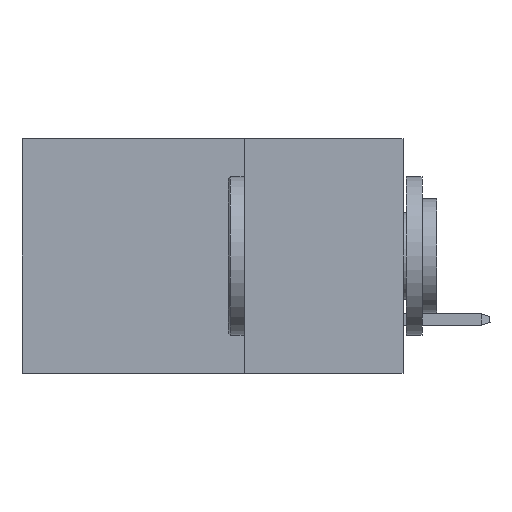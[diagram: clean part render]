
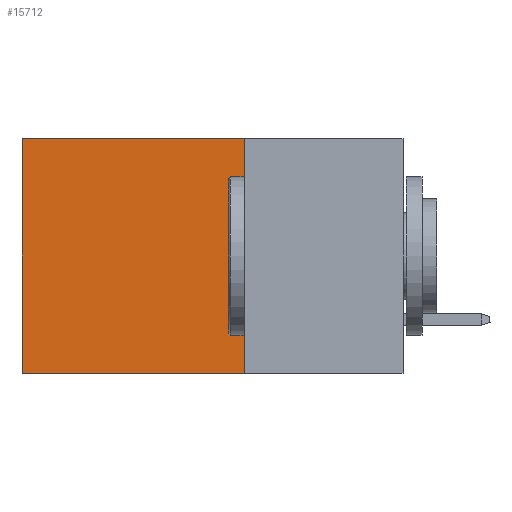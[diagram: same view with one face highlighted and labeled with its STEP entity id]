
A CAD part, left-side view. The second image highlights one B-rep face of the part: STEP entity #15712.
In plain terms, the highlighted planar face has unit normal (-1, 0, 0).
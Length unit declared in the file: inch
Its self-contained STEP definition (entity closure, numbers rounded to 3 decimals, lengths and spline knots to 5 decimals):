
#242 = LINE ( 'NONE', #23658, #15980 ) ;
#714 = VERTEX_POINT ( 'NONE', #7614 ) ;
#3190 = LINE ( 'NONE', #23038, #6921 ) ;
#3958 = VERTEX_POINT ( 'NONE', #17272 ) ;
#5454 = CARTESIAN_POINT ( 'NONE',  ( 0.2875, 0.25, 0. ) ) ;
#5765 = CARTESIAN_POINT ( 'NONE',  ( 0.2875, 0.25, 0. ) ) ;
#5849 = DIRECTION ( 'NONE',  ( 0., 0., -1. ) ) ;
#6921 = VECTOR ( 'NONE', #5849, 39.37008 ) ;
#7309 = EDGE_CURVE ( 'NONE', #17870, #3958, #10928, .T. ) ;
#7534 = EDGE_CURVE ( 'NONE', #3958, #714, #3190, .T. ) ;
#7614 = CARTESIAN_POINT ( 'NONE',  ( 0.2875, 0.6, -0.37 ) ) ;
#10928 = LINE ( 'NONE', #22209, #21706 ) ;
#11769 = EDGE_CURVE ( 'NONE', #17870, #19024, #21649, .T. ) ;
#11937 = ORIENTED_EDGE ( 'NONE', *, *, #7309, .T. ) ;
#12042 = ORIENTED_EDGE ( 'NONE', *, *, #7534, .T. ) ;
#12788 = DIRECTION ( 'NONE',  ( 1., 0., 0. ) ) ;
#14540 = AXIS2_PLACEMENT_3D ( 'NONE', #5765, #12788, #22839 ) ;
#15059 = CARTESIAN_POINT ( 'NONE',  ( 0.2875, 0.25, 0. ) ) ;
#15712 = ADVANCED_FACE ( 'NONE', ( #15724 ), #25125, .F. ) ;
#15724 = FACE_OUTER_BOUND ( 'NONE', #30210, .T. ) ;
#15980 = VECTOR ( 'NONE', #21356, 39.37008 ) ;
#16166 = EDGE_CURVE ( 'NONE', #19024, #714, #242, .T. ) ;
#17272 = CARTESIAN_POINT ( 'NONE',  ( 0.2875, 0.6, 0. ) ) ;
#17870 = VERTEX_POINT ( 'NONE', #15059 ) ;
#18013 = DIRECTION ( 'NONE',  ( 0., 1., 0. ) ) ;
#19024 = VERTEX_POINT ( 'NONE', #30000 ) ;
#19863 = ORIENTED_EDGE ( 'NONE', *, *, #11769, .F. ) ;
#21356 = DIRECTION ( 'NONE',  ( 0., 1., 0. ) ) ;
#21649 = LINE ( 'NONE', #5454, #21797 ) ;
#21706 = VECTOR ( 'NONE', #18013, 39.37008 ) ;
#21797 = VECTOR ( 'NONE', #24550, 39.37008 ) ;
#22209 = CARTESIAN_POINT ( 'NONE',  ( 0.2875, 0.25, 0. ) ) ;
#22839 = DIRECTION ( 'NONE',  ( 0., 0., -1. ) ) ;
#23038 = CARTESIAN_POINT ( 'NONE',  ( 0.2875, 0.6, 0. ) ) ;
#23658 = CARTESIAN_POINT ( 'NONE',  ( 0.2875, 0.25, -0.37 ) ) ;
#24550 = DIRECTION ( 'NONE',  ( 0., 0., -1. ) ) ;
#25125 = PLANE ( 'NONE',  #14540 ) ;
#25941 = ORIENTED_EDGE ( 'NONE', *, *, #16166, .F. ) ;
#30000 = CARTESIAN_POINT ( 'NONE',  ( 0.2875, 0.25, -0.37 ) ) ;
#30210 = EDGE_LOOP ( 'NONE', ( #12042, #25941, #19863, #11937 ) ) ;
